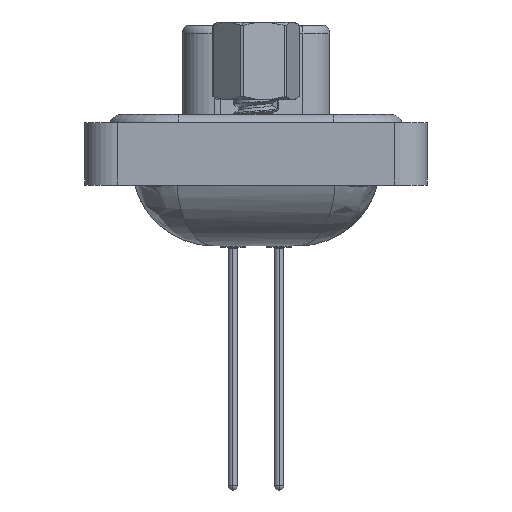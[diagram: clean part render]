
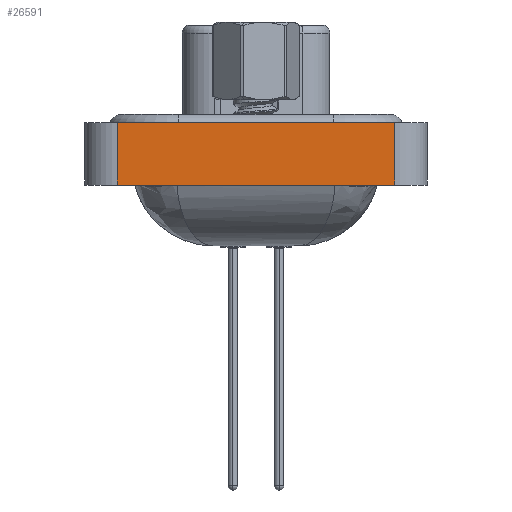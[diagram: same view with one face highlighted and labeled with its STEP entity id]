
A CAD part, left-side view. The second image highlights one B-rep face of the part: STEP entity #26591.
In plain terms, the highlighted planar face has unit normal (-1, 0, 0).
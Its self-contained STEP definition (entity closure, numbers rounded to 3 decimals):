
#1445 = CARTESIAN_POINT ( 'NONE',  ( -7.225, -8.55, 0.5 ) ) ;
#2130 = CARTESIAN_POINT ( 'NONE',  ( -7.225, -8.55, -3.35 ) ) ;
#2229 = EDGE_CURVE ( 'NONE', #3075, #22600, #16781, .T. ) ;
#3075 = VERTEX_POINT ( 'NONE', #21019 ) ;
#3309 = ORIENTED_EDGE ( 'NONE', *, *, #18180, .F. ) ;
#5568 = VERTEX_POINT ( 'NONE', #16517 ) ;
#5766 = DIRECTION ( 'NONE',  ( 0., 0., 1. ) ) ;
#6111 = DIRECTION ( 'NONE',  ( -1., 0., 0. ) ) ;
#6907 = ORIENTED_EDGE ( 'NONE', *, *, #2229, .T. ) ;
#9518 = ORIENTED_EDGE ( 'NONE', *, *, #24521, .F. ) ;
#9964 = CARTESIAN_POINT ( 'NONE',  ( -7.225, -8.55, -3.35 ) ) ;
#10129 = LINE ( 'NONE', #16458, #10473 ) ;
#10330 = FACE_OUTER_BOUND ( 'NONE', #11409, .T. ) ;
#10465 = LINE ( 'NONE', #1445, #16586 ) ;
#10473 = VECTOR ( 'NONE', #5766, 1000. ) ;
#11409 = EDGE_LOOP ( 'NONE', ( #25465, #9518, #3309, #6907 ) ) ;
#14180 = DIRECTION ( 'NONE',  ( 0., 0., 1. ) ) ;
#15089 = PLANE ( 'NONE',  #17790 ) ;
#16458 = CARTESIAN_POINT ( 'NONE',  ( -7.225, 8.55, -3.35 ) ) ;
#16517 = CARTESIAN_POINT ( 'NONE',  ( -7.225, 8.55, 0.5 ) ) ;
#16586 = VECTOR ( 'NONE', #18931, 1000. ) ;
#16781 = LINE ( 'NONE', #25522, #27019 ) ;
#17062 = DIRECTION ( 'NONE',  ( 0., -1., 0. ) ) ;
#17790 = AXIS2_PLACEMENT_3D ( 'NONE', #2130, #6111, #23573 ) ;
#18160 = LINE ( 'NONE', #9964, #24499 ) ;
#18180 = EDGE_CURVE ( 'NONE', #3075, #5568, #10129, .T. ) ;
#18810 = VERTEX_POINT ( 'NONE', #24819 ) ;
#18931 = DIRECTION ( 'NONE',  ( 0., -1., 0. ) ) ;
#20035 = EDGE_CURVE ( 'NONE', #22600, #18810, #18160, .T. ) ;
#21019 = CARTESIAN_POINT ( 'NONE',  ( -7.225, 8.55, -3.35 ) ) ;
#21548 = CARTESIAN_POINT ( 'NONE',  ( -7.225, -8.55, -3.35 ) ) ;
#22600 = VERTEX_POINT ( 'NONE', #21548 ) ;
#23573 = DIRECTION ( 'NONE',  ( 0., 0., 1. ) ) ;
#24499 = VECTOR ( 'NONE', #14180, 1000. ) ;
#24521 = EDGE_CURVE ( 'NONE', #5568, #18810, #10465, .T. ) ;
#24819 = CARTESIAN_POINT ( 'NONE',  ( -7.225, -8.55, 0.5 ) ) ;
#25465 = ORIENTED_EDGE ( 'NONE', *, *, #20035, .T. ) ;
#25522 = CARTESIAN_POINT ( 'NONE',  ( -7.225, -8.55, -3.35 ) ) ;
#26591 = ADVANCED_FACE ( 'NONE', ( #10330 ), #15089, .T. ) ;
#27019 = VECTOR ( 'NONE', #17062, 1000. ) ;
